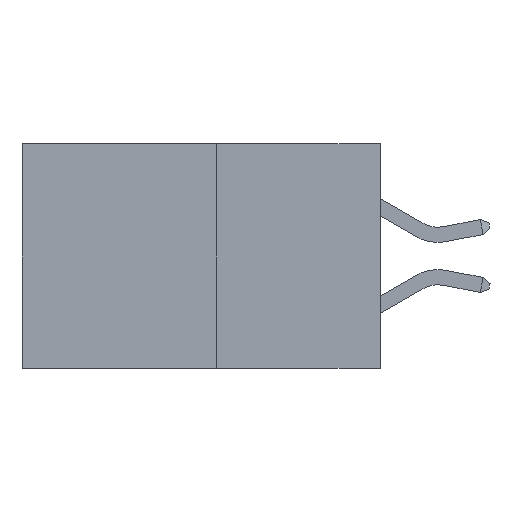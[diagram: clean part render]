
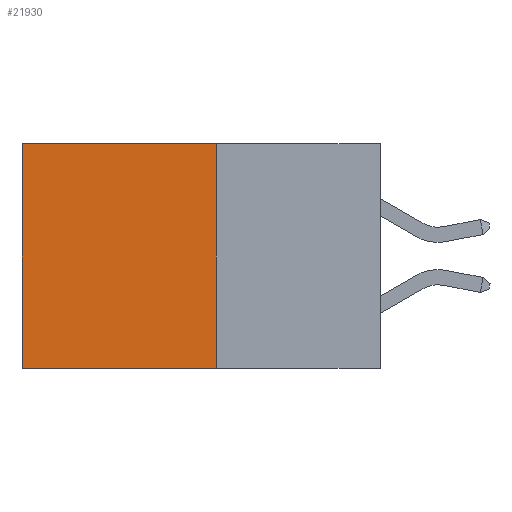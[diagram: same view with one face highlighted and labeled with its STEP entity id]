
A CAD part, left-side view. The second image highlights one B-rep face of the part: STEP entity #21930.
In plain terms, the highlighted planar face has unit normal (-1, 0, 0).
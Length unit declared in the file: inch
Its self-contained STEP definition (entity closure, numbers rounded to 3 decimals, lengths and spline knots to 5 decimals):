
#1248 = ORIENTED_EDGE ( 'NONE', *, *, #22276, .T. ) ;
#2642 = ORIENTED_EDGE ( 'NONE', *, *, #24750, .T. ) ;
#2870 = CARTESIAN_POINT ( 'NONE',  ( 0.277, 0.27, -0.37 ) ) ;
#5562 = DIRECTION ( 'NONE',  ( 0., 0., -1. ) ) ;
#6182 = LINE ( 'NONE', #30550, #31443 ) ;
#6361 = FACE_OUTER_BOUND ( 'NONE', #30763, .T. ) ;
#7822 = VERTEX_POINT ( 'NONE', #24715 ) ;
#7976 = VERTEX_POINT ( 'NONE', #10639 ) ;
#9326 = DIRECTION ( 'NONE',  ( 0., 1., 0. ) ) ;
#10191 = AXIS2_PLACEMENT_3D ( 'NONE', #15391, #20251, #5562 ) ;
#10384 = VERTEX_POINT ( 'NONE', #19048 ) ;
#10385 = DIRECTION ( 'NONE',  ( 0., 0., -1. ) ) ;
#10639 = CARTESIAN_POINT ( 'NONE',  ( 0.277, 0.27, -0.37 ) ) ;
#11004 = ORIENTED_EDGE ( 'NONE', *, *, #17054, .F. ) ;
#12657 = CARTESIAN_POINT ( 'NONE',  ( 0.277, 0.27, -0.37 ) ) ;
#14105 = EDGE_CURVE ( 'NONE', #7976, #20824, #20730, .T. ) ;
#14275 = VECTOR ( 'NONE', #22410, 39.37008 ) ;
#14859 = CARTESIAN_POINT ( 'NONE',  ( 0.277, 0.59, -0.37 ) ) ;
#15195 = ORIENTED_EDGE ( 'NONE', *, *, #14105, .F. ) ;
#15250 = LINE ( 'NONE', #19067, #27414 ) ;
#15391 = CARTESIAN_POINT ( 'NONE',  ( 0.277, 0.27, -0.37 ) ) ;
#17054 = EDGE_CURVE ( 'NONE', #10384, #7976, #24331, .T. ) ;
#17860 = VECTOR ( 'NONE', #10385, 39.37008 ) ;
#19048 = CARTESIAN_POINT ( 'NONE',  ( 0.277, 0.27, 0. ) ) ;
#19067 = CARTESIAN_POINT ( 'NONE',  ( 0.277, 0.27, 0. ) ) ;
#20251 = DIRECTION ( 'NONE',  ( 1., 0., 0. ) ) ;
#20730 = LINE ( 'NONE', #12657, #14275 ) ;
#20824 = VERTEX_POINT ( 'NONE', #14859 ) ;
#21930 = ADVANCED_FACE ( 'NONE', ( #6361 ), #27515, .F. ) ;
#22276 = EDGE_CURVE ( 'NONE', #10384, #7822, #15250, .T. ) ;
#22410 = DIRECTION ( 'NONE',  ( 0., 1., 0. ) ) ;
#24331 = LINE ( 'NONE', #2870, #17860 ) ;
#24715 = CARTESIAN_POINT ( 'NONE',  ( 0.277, 0.59, 0. ) ) ;
#24750 = EDGE_CURVE ( 'NONE', #7822, #20824, #6182, .T. ) ;
#27414 = VECTOR ( 'NONE', #9326, 39.37008 ) ;
#27515 = PLANE ( 'NONE',  #10191 ) ;
#30550 = CARTESIAN_POINT ( 'NONE',  ( 0.277, 0.59, -0.37 ) ) ;
#30644 = DIRECTION ( 'NONE',  ( 0., 0., -1. ) ) ;
#30763 = EDGE_LOOP ( 'NONE', ( #2642, #15195, #11004, #1248 ) ) ;
#31443 = VECTOR ( 'NONE', #30644, 39.37008 ) ;
